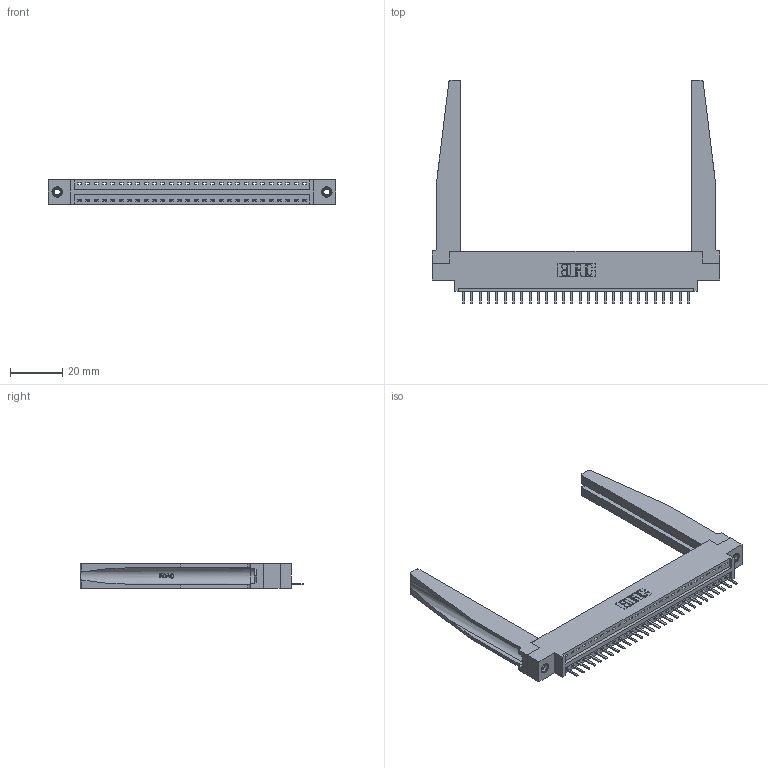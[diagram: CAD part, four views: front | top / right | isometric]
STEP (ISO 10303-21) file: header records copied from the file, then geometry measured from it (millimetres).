
FILE_DESCRIPTION (( 'STEP AP203' ), '1' );
FILE_NAME ('346-028-520-678.STEP', '2022-05-06T06:20:27', ( '' ), ( '' ), 'SwSTEP 2.0', 'SolidWorks 2020', '' );
FILE_SCHEMA (( 'CONFIG_CONTROL_DESIGN' ));
Length unit declared in the file: inch
Products named in the file (5): 345-250-001_345-250-001-102; 346-028-520-678; 345-292-001_345-293-120; 346 Part_0.170 Offset - 0.156 Dia-TH; 346-220-078_345-220-078
Assembly tree (33 placements, depth 2):
  346-028-520-678
    346 Part_0.170 Offset - 0.156 Dia-TH
    345-292-001_345-293-120  x28
    346-220-078_345-220-078  x2
    345-250-001_345-250-001-102  x2
Bounding box: 109.47 x 85.29 x 9.4 mm (x, y, z)
Volume: 17038.2 mm3; surface area: 18973.2 mm2
Topology: 33 solids, 33 shells, 2110 faces, 6137 edges, 4006 vertices
Faces by surface type: plane 1412, cylinder 646, bspline 36, cone 12, torus 4
Entity records: 24672 total; most frequent: CARTESIAN_POINT 5161, ORIENTED_EDGE 3998, DIRECTION 3541, EDGE_CURVE 1999, VECTOR 1657, LINE 1657, VERTEX_POINT 1324, AXIS2_PLACEMENT_3D 942
